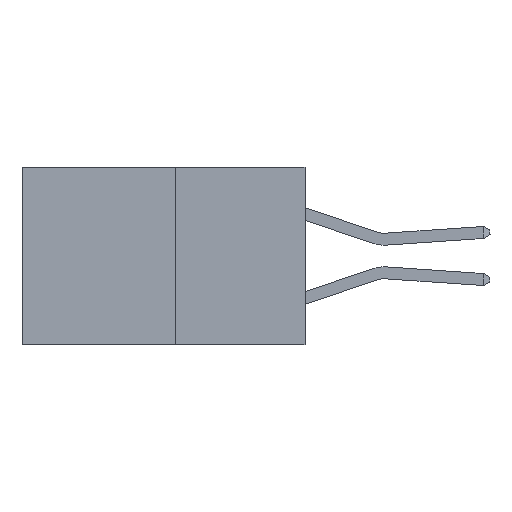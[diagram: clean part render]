
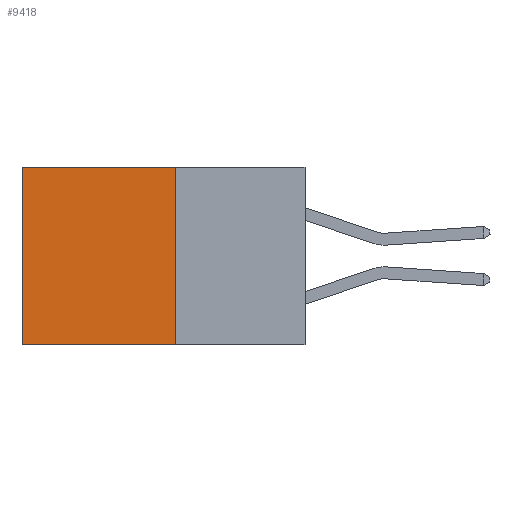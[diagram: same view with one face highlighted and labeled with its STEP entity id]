
A CAD part, left-side view. The second image highlights one B-rep face of the part: STEP entity #9418.
In plain terms, the highlighted planar face has unit normal (-1, 0, 0).
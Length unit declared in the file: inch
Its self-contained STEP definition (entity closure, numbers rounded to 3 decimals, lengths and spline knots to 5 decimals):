
#117 = LINE ( 'NONE', #5956, #18644 ) ;
#525 = ORIENTED_EDGE ( 'NONE', *, *, #16120, .T. ) ;
#897 = DIRECTION ( 'NONE',  ( 0., 0., -1. ) ) ;
#1357 = EDGE_CURVE ( 'NONE', #11081, #8125, #4860, .T. ) ;
#1442 = CARTESIAN_POINT ( 'NONE',  ( 0.277, 0.27, -0.37 ) ) ;
#1715 = ORIENTED_EDGE ( 'NONE', *, *, #8114, .T. ) ;
#2324 = CARTESIAN_POINT ( 'NONE',  ( 0.277, 0.27, -0.37 ) ) ;
#3367 = DIRECTION ( 'NONE',  ( 0., 1., 0. ) ) ;
#4386 = CARTESIAN_POINT ( 'NONE',  ( 0.277, 0.27, 0. ) ) ;
#4860 = LINE ( 'NONE', #1442, #12220 ) ;
#4865 = FACE_OUTER_BOUND ( 'NONE', #13190, .T. ) ;
#5380 = LINE ( 'NONE', #12819, #12278 ) ;
#5956 = CARTESIAN_POINT ( 'NONE',  ( 0.277, 0.27, -0.37 ) ) ;
#6455 = VERTEX_POINT ( 'NONE', #17412 ) ;
#6566 = AXIS2_PLACEMENT_3D ( 'NONE', #2324, #9688, #897 ) ;
#8114 = EDGE_CURVE ( 'NONE', #6455, #8125, #5380, .T. ) ;
#8125 = VERTEX_POINT ( 'NONE', #14323 ) ;
#8432 = LINE ( 'NONE', #4386, #16217 ) ;
#9418 = ADVANCED_FACE ( 'NONE', ( #4865 ), #18394, .F. ) ;
#9688 = DIRECTION ( 'NONE',  ( 1., 0., 0. ) ) ;
#11081 = VERTEX_POINT ( 'NONE', #13941 ) ;
#12042 = VERTEX_POINT ( 'NONE', #18908 ) ;
#12220 = VECTOR ( 'NONE', #3367, 39.37008 ) ;
#12278 = VECTOR ( 'NONE', #18624, 39.37008 ) ;
#12819 = CARTESIAN_POINT ( 'NONE',  ( 0.277, 0.59, -0.37 ) ) ;
#13190 = EDGE_LOOP ( 'NONE', ( #1715, #13833, #18140, #525 ) ) ;
#13833 = ORIENTED_EDGE ( 'NONE', *, *, #1357, .F. ) ;
#13941 = CARTESIAN_POINT ( 'NONE',  ( 0.277, 0.27, -0.37 ) ) ;
#14323 = CARTESIAN_POINT ( 'NONE',  ( 0.277, 0.59, -0.37 ) ) ;
#16120 = EDGE_CURVE ( 'NONE', #12042, #6455, #8432, .T. ) ;
#16166 = DIRECTION ( 'NONE',  ( 0., 0., -1. ) ) ;
#16217 = VECTOR ( 'NONE', #18914, 39.37008 ) ;
#17150 = EDGE_CURVE ( 'NONE', #12042, #11081, #117, .T. ) ;
#17412 = CARTESIAN_POINT ( 'NONE',  ( 0.277, 0.59, 0. ) ) ;
#18140 = ORIENTED_EDGE ( 'NONE', *, *, #17150, .F. ) ;
#18394 = PLANE ( 'NONE',  #6566 ) ;
#18624 = DIRECTION ( 'NONE',  ( 0., 0., -1. ) ) ;
#18644 = VECTOR ( 'NONE', #16166, 39.37008 ) ;
#18908 = CARTESIAN_POINT ( 'NONE',  ( 0.277, 0.27, 0. ) ) ;
#18914 = DIRECTION ( 'NONE',  ( 0., 1., 0. ) ) ;
